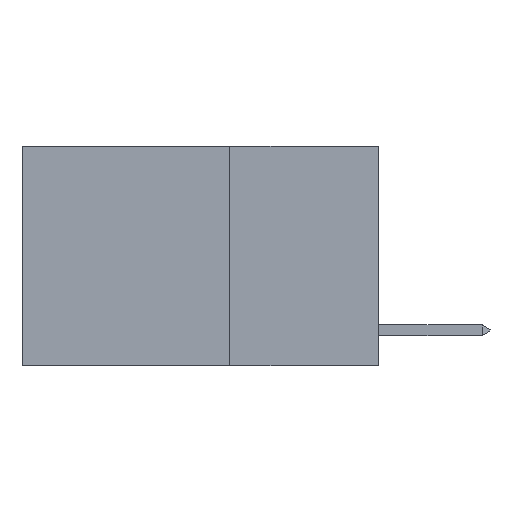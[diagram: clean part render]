
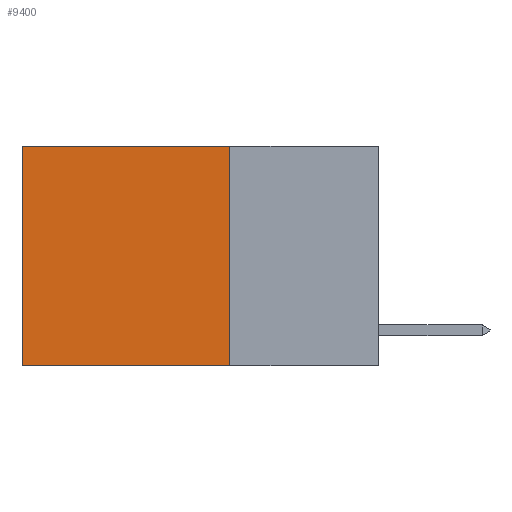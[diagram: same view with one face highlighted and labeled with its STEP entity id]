
A CAD part, left-side view. The second image highlights one B-rep face of the part: STEP entity #9400.
In plain terms, the highlighted planar face has unit normal (-1, 0, 0).
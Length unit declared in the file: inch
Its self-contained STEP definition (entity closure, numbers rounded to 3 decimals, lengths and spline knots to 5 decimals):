
#610 = CARTESIAN_POINT ( 'NONE',  ( 0.2625, 0.25, 0. ) ) ;
#695 = VERTEX_POINT ( 'NONE', #6282 ) ;
#1060 = CARTESIAN_POINT ( 'NONE',  ( 0.2625, 0.25, -0.37 ) ) ;
#2874 = LINE ( 'NONE', #1060, #22314 ) ;
#4464 = VECTOR ( 'NONE', #11409, 39.37008 ) ;
#6282 = CARTESIAN_POINT ( 'NONE',  ( 0.2625, 0.6, -0.37 ) ) ;
#6554 = CARTESIAN_POINT ( 'NONE',  ( 0.2625, 0.25, -0.37 ) ) ;
#8054 = LINE ( 'NONE', #13640, #4464 ) ;
#8285 = DIRECTION ( 'NONE',  ( 0., 0., -1. ) ) ;
#8413 = CARTESIAN_POINT ( 'NONE',  ( 0.2625, 0.25, 0. ) ) ;
#9155 = VERTEX_POINT ( 'NONE', #12703 ) ;
#9400 = ADVANCED_FACE ( 'NONE', ( #15922 ), #19923, .F. ) ;
#10842 = DIRECTION ( 'NONE',  ( 0., 1., 0. ) ) ;
#11409 = DIRECTION ( 'NONE',  ( 0., 1., 0. ) ) ;
#12374 = EDGE_CURVE ( 'NONE', #17326, #695, #2874, .T. ) ;
#12703 = CARTESIAN_POINT ( 'NONE',  ( 0.2625, 0.25, 0. ) ) ;
#13016 = ORIENTED_EDGE ( 'NONE', *, *, #19905, .F. ) ;
#13069 = VECTOR ( 'NONE', #20215, 39.37008 ) ;
#13332 = ORIENTED_EDGE ( 'NONE', *, *, #12374, .F. ) ;
#13640 = CARTESIAN_POINT ( 'NONE',  ( 0.2625, 0.25, 0. ) ) ;
#14378 = DIRECTION ( 'NONE',  ( 1., 0., 0. ) ) ;
#15497 = ORIENTED_EDGE ( 'NONE', *, *, #25274, .T. ) ;
#15674 = LINE ( 'NONE', #17608, #19573 ) ;
#15922 = FACE_OUTER_BOUND ( 'NONE', #20689, .T. ) ;
#17326 = VERTEX_POINT ( 'NONE', #6554 ) ;
#17608 = CARTESIAN_POINT ( 'NONE',  ( 0.2625, 0.6, 0. ) ) ;
#17909 = CARTESIAN_POINT ( 'NONE',  ( 0.2625, 0.6, 0. ) ) ;
#18256 = EDGE_CURVE ( 'NONE', #22459, #695, #15674, .T. ) ;
#18532 = LINE ( 'NONE', #610, #13069 ) ;
#19573 = VECTOR ( 'NONE', #24020, 39.37008 ) ;
#19905 = EDGE_CURVE ( 'NONE', #9155, #17326, #18532, .T. ) ;
#19923 = PLANE ( 'NONE',  #23846 ) ;
#20215 = DIRECTION ( 'NONE',  ( 0., 0., -1. ) ) ;
#20420 = ORIENTED_EDGE ( 'NONE', *, *, #18256, .T. ) ;
#20689 = EDGE_LOOP ( 'NONE', ( #20420, #13332, #13016, #15497 ) ) ;
#22314 = VECTOR ( 'NONE', #10842, 39.37008 ) ;
#22459 = VERTEX_POINT ( 'NONE', #17909 ) ;
#23846 = AXIS2_PLACEMENT_3D ( 'NONE', #8413, #14378, #8285 ) ;
#24020 = DIRECTION ( 'NONE',  ( 0., 0., -1. ) ) ;
#25274 = EDGE_CURVE ( 'NONE', #9155, #22459, #8054, .T. ) ;
